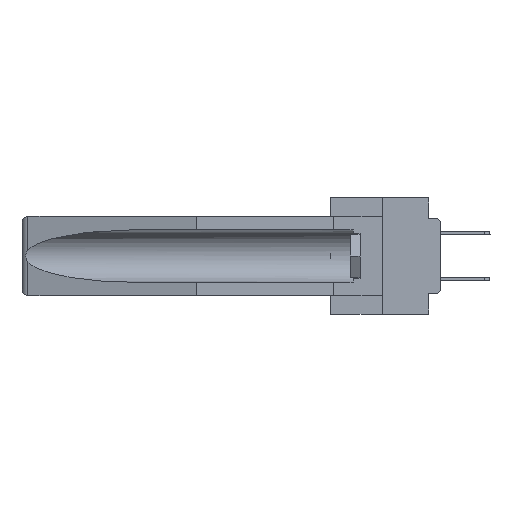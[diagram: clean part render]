
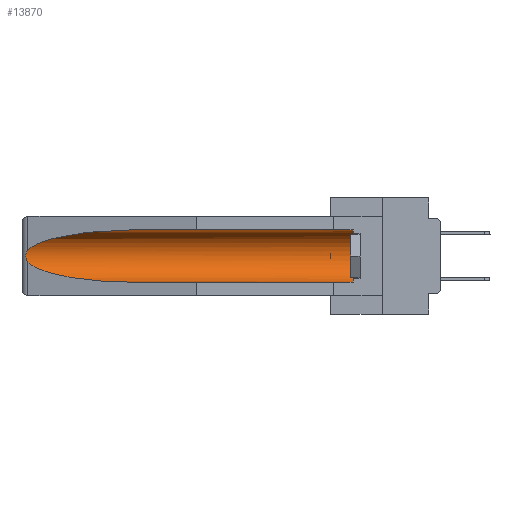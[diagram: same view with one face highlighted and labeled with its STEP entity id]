
A CAD part, left-side view. The second image highlights one B-rep face of the part: STEP entity #13870.
In plain terms, the highlighted cylindrical face has radius 2.857 mm (diameter 5.715 mm), a partial arc.
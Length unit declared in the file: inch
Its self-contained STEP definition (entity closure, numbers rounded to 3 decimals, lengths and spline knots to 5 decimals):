
#2476 = EDGE_CURVE ( 'NONE', #15215, #17262, #26230, .T. ) ;
#2584 = LINE ( 'NONE', #37061, #5862 ) ;
#2586 = ORIENTED_EDGE ( 'NONE', *, *, #3617, .T. ) ;
#2918 = CARTESIAN_POINT ( 'NONE',  ( 0.25451, 1.48313, -0.24835 ) ) ;
#3329 = CARTESIAN_POINT ( 'NONE',  ( 0.155, 1.07973, -0.284 ) ) ;
#3617 = EDGE_CURVE ( 'NONE', #9666, #19780, #28163, .T. ) ;
#5422 = CARTESIAN_POINT ( 'NONE',  ( 0.26537, 1.52718, -0.19328 ) ) ;
#5862 = VECTOR ( 'NONE', #5865, 39.37008 ) ;
#5865 = DIRECTION ( 'NONE',  ( 0., 1., 0. ) ) ;
#6486 = CARTESIAN_POINT ( 'NONE',  ( 0.155, 1.07973, -0.059 ) ) ;
#7402 = VERTEX_POINT ( 'NONE', #3329 ) ;
#7890 = CARTESIAN_POINT ( 'NONE',  ( 0.26537, 1.52718, -0.14972 ) ) ;
#8959 = AXIS2_PLACEMENT_3D ( 'NONE', #12172, #37646, #9498 ) ;
#9498 = DIRECTION ( 'NONE',  ( 0., 0., 1. ) ) ;
#9593 = CIRCLE ( 'NONE', #8959, 0.1125 ) ;
#9666 = VERTEX_POINT ( 'NONE', #7890 ) ;
#10009 = CARTESIAN_POINT ( 'NONE',  ( 0.25451, 1.48313, -0.09465 ) ) ;
#10987 = CARTESIAN_POINT ( 'NONE',  ( 0.155, 0.126, -0.059 ) ) ;
#11162 = CARTESIAN_POINT ( 'NONE',  ( 0.26597, 1.5296, -0.19026 ) ) ;
#11169 = EDGE_CURVE ( 'NONE', #31318, #7402, #2584, .T. ) ;
#12172 = CARTESIAN_POINT ( 'NONE',  ( 0.155, 0.126, -0.1715 ) ) ;
#12741 = CARTESIAN_POINT ( 'NONE',  ( 0.155, 1.07973, -0.284 ) ) ;
#13061 = ORIENTED_EDGE ( 'NONE', *, *, #38819, .T. ) ;
#13870 = ADVANCED_FACE ( 'NONE', ( #29031 ), #22875, .F. ) ;
#14014 = DIRECTION ( 'NONE',  ( 0., 1., 0. ) ) ;
#14182 = EDGE_LOOP ( 'NONE', ( #37244, #2586, #26860, #33927, #13061, #19823 ) ) ;
#15215 = VERTEX_POINT ( 'NONE', #10987 ) ;
#16317 = CARTESIAN_POINT ( 'NONE',  ( 0.155, -0.30754, -0.1715 ) ) ;
#16405 = EDGE_CURVE ( 'NONE', #19780, #7402, #18197, .T. ) ;
#16504 = DIRECTION ( 'NONE',  ( 0., 0., 1. ) ) ;
#17262 = VERTEX_POINT ( 'NONE', #6486 ) ;
#18127 = CARTESIAN_POINT ( 'NONE',  ( 0.2673, 1.5327, -0.16383 ) ) ;
#18197 =( BOUNDED_CURVE ( )  B_SPLINE_CURVE ( 3, ( #31029, #2918, #27963, #12741 ),
 .UNSPECIFIED., .F., .F. ) 
 B_SPLINE_CURVE_WITH_KNOTS ( ( 4, 4 ),
 ( 0.1948, 1.5708 ),
 .UNSPECIFIED. ) 
 CURVE ( )  GEOMETRIC_REPRESENTATION_ITEM ( )  RATIONAL_B_SPLINE_CURVE ( ( 1., 0.848, 0.848, 1. ) ) 
 REPRESENTATION_ITEM ( '' )  );
#18252 = CARTESIAN_POINT ( 'NONE',  ( 0.26537, 1.52718, -0.19328 ) ) ;
#18634 = AXIS2_PLACEMENT_3D ( 'NONE', #16317, #14014, #16504 ) ;
#19780 = VERTEX_POINT ( 'NONE', #18252 ) ;
#19823 = ORIENTED_EDGE ( 'NONE', *, *, #2476, .T. ) ;
#22382 =( BOUNDED_CURVE ( )  B_SPLINE_CURVE ( 3, ( #37751, #34874, #10009, #22517 ),
 .UNSPECIFIED., .F., .F. ) 
 B_SPLINE_CURVE_WITH_KNOTS ( ( 4, 4 ),
 ( 4.71239, 6.08839 ),
 .UNSPECIFIED. ) 
 CURVE ( )  GEOMETRIC_REPRESENTATION_ITEM ( )  RATIONAL_B_SPLINE_CURVE ( ( 1., 0.848, 0.848, 1. ) ) 
 REPRESENTATION_ITEM ( '' )  );
#22503 = VECTOR ( 'NONE', #29524, 39.37008 ) ;
#22517 = CARTESIAN_POINT ( 'NONE',  ( 0.26537, 1.52718, -0.14972 ) ) ;
#22875 = CYLINDRICAL_SURFACE ( 'NONE', #18634, 0.1125 ) ;
#24098 = CARTESIAN_POINT ( 'NONE',  ( 0.2673, 1.53269, -0.17917 ) ) ;
#25089 = CARTESIAN_POINT ( 'NONE',  ( 0.155, 0.126, -0.284 ) ) ;
#26230 = LINE ( 'NONE', #35299, #22503 ) ;
#26781 = CARTESIAN_POINT ( 'NONE',  ( 0.2675, 1.53308, -0.17534 ) ) ;
#26860 = ORIENTED_EDGE ( 'NONE', *, *, #16405, .T. ) ;
#27162 = CARTESIAN_POINT ( 'NONE',  ( 0.26597, 1.52961, -0.15275 ) ) ;
#27963 = CARTESIAN_POINT ( 'NONE',  ( 0.21114, 1.30732, -0.284 ) ) ;
#28163 = B_SPLINE_CURVE_WITH_KNOTS ( 'NONE', 3,
 ( #33973, #27162, #39326, #18127, #39716, #26781, #24098, #36648, #11162, #5422 ),
 .UNSPECIFIED., .F., .F.,
 ( 4, 2, 2, 2, 4 ),
 ( 0., 0.00029, 0.00058, 0.00087, 0.00117 ),
 .UNSPECIFIED. ) ;
#29031 = FACE_OUTER_BOUND ( 'NONE', #14182, .T. ) ;
#29524 = DIRECTION ( 'NONE',  ( 0., 1., 0. ) ) ;
#31029 = CARTESIAN_POINT ( 'NONE',  ( 0.26537, 1.52718, -0.19328 ) ) ;
#31318 = VERTEX_POINT ( 'NONE', #25089 ) ;
#33927 = ORIENTED_EDGE ( 'NONE', *, *, #11169, .F. ) ;
#33973 = CARTESIAN_POINT ( 'NONE',  ( 0.26537, 1.52718, -0.14972 ) ) ;
#34714 = EDGE_CURVE ( 'NONE', #17262, #9666, #22382, .T. ) ;
#34874 = CARTESIAN_POINT ( 'NONE',  ( 0.21114, 1.30732, -0.059 ) ) ;
#35299 = CARTESIAN_POINT ( 'NONE',  ( 0.155, -0.30754, -0.059 ) ) ;
#36648 = CARTESIAN_POINT ( 'NONE',  ( 0.26655, 1.53094, -0.18657 ) ) ;
#37061 = CARTESIAN_POINT ( 'NONE',  ( 0.155, -0.30754, -0.284 ) ) ;
#37244 = ORIENTED_EDGE ( 'NONE', *, *, #34714, .T. ) ;
#37646 = DIRECTION ( 'NONE',  ( 0., -1., 0. ) ) ;
#37751 = CARTESIAN_POINT ( 'NONE',  ( 0.155, 1.07973, -0.059 ) ) ;
#38819 = EDGE_CURVE ( 'NONE', #31318, #15215, #9593, .T. ) ;
#39326 = CARTESIAN_POINT ( 'NONE',  ( 0.26654, 1.53092, -0.15636 ) ) ;
#39716 = CARTESIAN_POINT ( 'NONE',  ( 0.2675, 1.53308, -0.16763 ) ) ;
